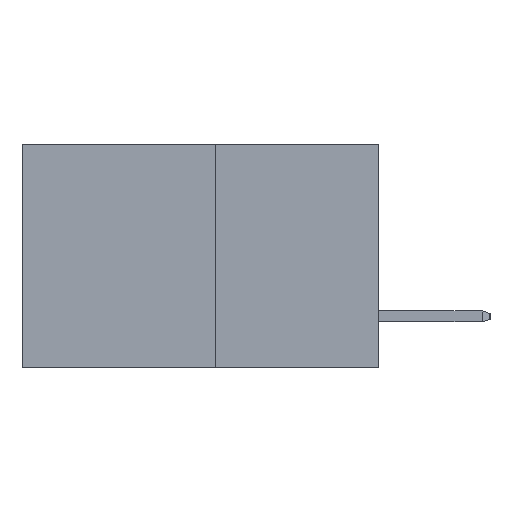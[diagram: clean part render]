
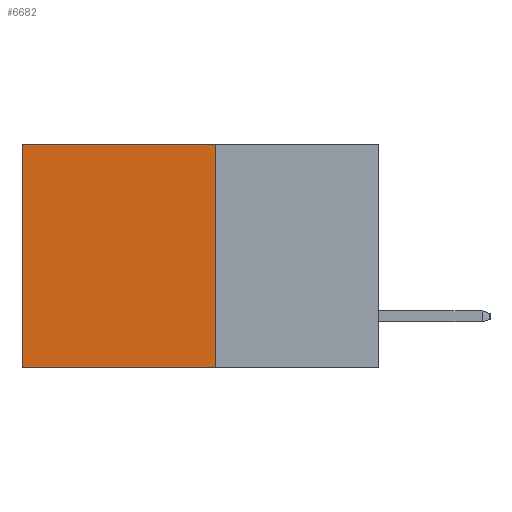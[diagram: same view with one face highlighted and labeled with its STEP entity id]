
A CAD part, left-side view. The second image highlights one B-rep face of the part: STEP entity #6682.
In plain terms, the highlighted planar face has unit normal (-1, 0, 0).
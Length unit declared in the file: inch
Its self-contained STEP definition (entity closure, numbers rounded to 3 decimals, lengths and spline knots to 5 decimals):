
#420 = DIRECTION ( 'NONE',  ( 0., 0., -1. ) ) ;
#597 = FACE_OUTER_BOUND ( 'NONE', #1211, .T. ) ;
#1129 = VERTEX_POINT ( 'NONE', #7660 ) ;
#1211 = EDGE_LOOP ( 'NONE', ( #2142, #5303, #1987, #8268 ) ) ;
#1639 = PLANE ( 'NONE',  #7096 ) ;
#1777 = EDGE_CURVE ( 'NONE', #9218, #1129, #9182, .T. ) ;
#1940 = VERTEX_POINT ( 'NONE', #5438 ) ;
#1987 = ORIENTED_EDGE ( 'NONE', *, *, #4745, .F. ) ;
#2142 = ORIENTED_EDGE ( 'NONE', *, *, #6008, .T. ) ;
#3828 = VECTOR ( 'NONE', #10275, 39.37008 ) ;
#3972 = DIRECTION ( 'NONE',  ( 0., 1., 0. ) ) ;
#4745 = EDGE_CURVE ( 'NONE', #9432, #9218, #7954, .T. ) ;
#5303 = ORIENTED_EDGE ( 'NONE', *, *, #1777, .F. ) ;
#5438 = CARTESIAN_POINT ( 'NONE',  ( 0.277, 0.59, 0. ) ) ;
#6008 = EDGE_CURVE ( 'NONE', #1940, #1129, #10927, .T. ) ;
#6040 = CARTESIAN_POINT ( 'NONE',  ( 0.277, 0.27, 0. ) ) ;
#6682 = ADVANCED_FACE ( 'NONE', ( #597 ), #1639, .F. ) ;
#7096 = AXIS2_PLACEMENT_3D ( 'NONE', #10975, #10973, #7124 ) ;
#7124 = DIRECTION ( 'NONE',  ( 0., 0., -1. ) ) ;
#7520 = LINE ( 'NONE', #11030, #10181 ) ;
#7660 = CARTESIAN_POINT ( 'NONE',  ( 0.277, 0.59, -0.37 ) ) ;
#7954 = LINE ( 'NONE', #8733, #12967 ) ;
#8230 = VECTOR ( 'NONE', #420, 39.37008 ) ;
#8268 = ORIENTED_EDGE ( 'NONE', *, *, #10477, .T. ) ;
#8733 = CARTESIAN_POINT ( 'NONE',  ( 0.277, 0.27, -0.37 ) ) ;
#9182 = LINE ( 'NONE', #10318, #3828 ) ;
#9218 = VERTEX_POINT ( 'NONE', #10209 ) ;
#9432 = VERTEX_POINT ( 'NONE', #6040 ) ;
#10181 = VECTOR ( 'NONE', #3972, 39.37008 ) ;
#10209 = CARTESIAN_POINT ( 'NONE',  ( 0.277, 0.27, -0.37 ) ) ;
#10275 = DIRECTION ( 'NONE',  ( 0., 1., 0. ) ) ;
#10318 = CARTESIAN_POINT ( 'NONE',  ( 0.277, 0.27, -0.37 ) ) ;
#10477 = EDGE_CURVE ( 'NONE', #9432, #1940, #7520, .T. ) ;
#10927 = LINE ( 'NONE', #11432, #8230 ) ;
#10973 = DIRECTION ( 'NONE',  ( 1., 0., 0. ) ) ;
#10975 = CARTESIAN_POINT ( 'NONE',  ( 0.277, 0.27, -0.37 ) ) ;
#11030 = CARTESIAN_POINT ( 'NONE',  ( 0.277, 0.27, 0. ) ) ;
#11041 = DIRECTION ( 'NONE',  ( 0., 0., -1. ) ) ;
#11432 = CARTESIAN_POINT ( 'NONE',  ( 0.277, 0.59, -0.37 ) ) ;
#12967 = VECTOR ( 'NONE', #11041, 39.37008 ) ;
